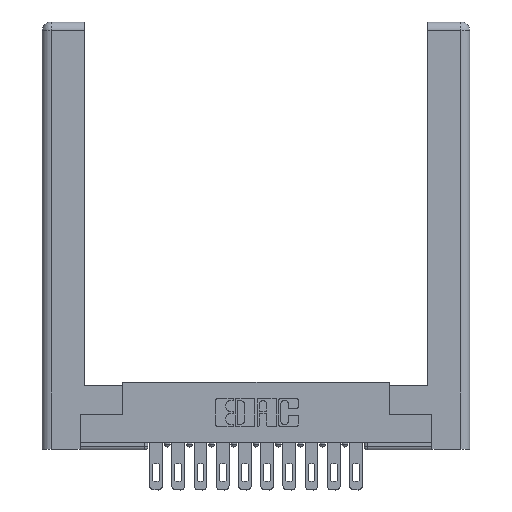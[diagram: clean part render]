
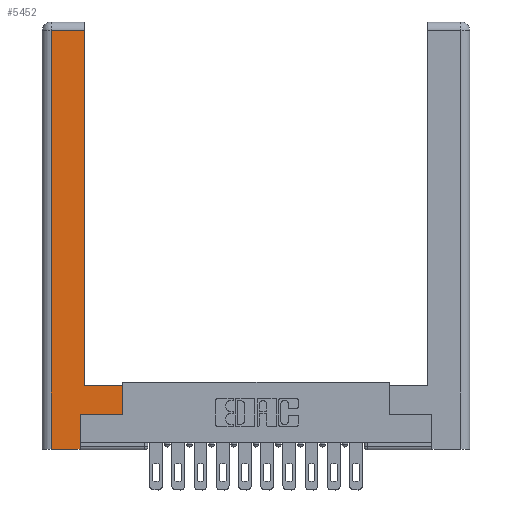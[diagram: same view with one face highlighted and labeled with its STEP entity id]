
A CAD part, top view. The second image highlights one B-rep face of the part: STEP entity #5452.
In plain terms, the highlighted planar face has unit normal (0, 0, 1).
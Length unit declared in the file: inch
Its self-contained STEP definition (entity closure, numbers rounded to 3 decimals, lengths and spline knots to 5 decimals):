
#91 = VERTEX_POINT ( 'NONE', #697 ) ;
#570 = VECTOR ( 'NONE', #2450, 39.37008 ) ;
#615 = DIRECTION ( 'NONE',  ( -1., 0., 0. ) ) ;
#697 = CARTESIAN_POINT ( 'NONE',  ( 0.0615, 2.94, 0. ) ) ;
#889 = CARTESIAN_POINT ( 'NONE',  ( 0.565, 0.45, 0. ) ) ;
#1073 = EDGE_CURVE ( 'NONE', #10897, #91, #7001, .T. ) ;
#1170 = VECTOR ( 'NONE', #13266, 39.37008 ) ;
#1200 = DIRECTION ( 'NONE',  ( -1., 0., 0. ) ) ;
#1414 = CARTESIAN_POINT ( 'NONE',  ( 0.295, 3., 0. ) ) ;
#1536 = ORIENTED_EDGE ( 'NONE', *, *, #7700, .T. ) ;
#1684 = FACE_OUTER_BOUND ( 'NONE', #1974, .T. ) ;
#1974 = EDGE_LOOP ( 'NONE', ( #2211, #2026, #6746, #7909, #13455, #1536, #10205, #5857 ) ) ;
#2026 = ORIENTED_EDGE ( 'NONE', *, *, #1073, .T. ) ;
#2033 = LINE ( 'NONE', #8176, #11463 ) ;
#2171 = VECTOR ( 'NONE', #4620, 39.37008 ) ;
#2211 = ORIENTED_EDGE ( 'NONE', *, *, #7150, .T. ) ;
#2450 = DIRECTION ( 'NONE',  ( -1., 0., 0. ) ) ;
#2715 = CARTESIAN_POINT ( 'NONE',  ( 0.295, 2.94, 0. ) ) ;
#2726 = VERTEX_POINT ( 'NONE', #13794 ) ;
#4239 = DIRECTION ( 'NONE',  ( 0., -1., 0. ) ) ;
#4620 = DIRECTION ( 'NONE',  ( 1., 0., 0. ) ) ;
#4949 = CARTESIAN_POINT ( 'NONE',  ( 0.265, 0., 0. ) ) ;
#5452 = ADVANCED_FACE ( 'NONE', ( #1684 ), #7741, .F. ) ;
#5709 = VERTEX_POINT ( 'NONE', #13240 ) ;
#5855 = CARTESIAN_POINT ( 'NONE',  ( 0.265, 0., 0. ) ) ;
#5857 = ORIENTED_EDGE ( 'NONE', *, *, #6094, .T. ) ;
#5921 = CARTESIAN_POINT ( 'NONE',  ( 0.0615, 2.94, 0. ) ) ;
#6094 = EDGE_CURVE ( 'NONE', #5709, #6208, #2033, .T. ) ;
#6208 = VERTEX_POINT ( 'NONE', #12914 ) ;
#6320 = VERTEX_POINT ( 'NONE', #14622 ) ;
#6377 = LINE ( 'NONE', #13341, #1170 ) ;
#6715 = VERTEX_POINT ( 'NONE', #4949 ) ;
#6746 = ORIENTED_EDGE ( 'NONE', *, *, #8407, .T. ) ;
#6782 = VECTOR ( 'NONE', #10089, 39.37008 ) ;
#7001 = LINE ( 'NONE', #5921, #570 ) ;
#7150 = EDGE_CURVE ( 'NONE', #6208, #10897, #10617, .T. ) ;
#7404 = EDGE_CURVE ( 'NONE', #9547, #6715, #13967, .T. ) ;
#7700 = EDGE_CURVE ( 'NONE', #2726, #6320, #6377, .T. ) ;
#7741 = PLANE ( 'NONE',  #7768 ) ;
#7768 = AXIS2_PLACEMENT_3D ( 'NONE', #8889, #13415, #615 ) ;
#7909 = ORIENTED_EDGE ( 'NONE', *, *, #7404, .T. ) ;
#8176 = CARTESIAN_POINT ( 'NONE',  ( 0.295, 0.45, 0. ) ) ;
#8407 = EDGE_CURVE ( 'NONE', #91, #9547, #12298, .T. ) ;
#8889 = CARTESIAN_POINT ( 'NONE',  ( 0., 0., 0. ) ) ;
#9465 = DIRECTION ( 'NONE',  ( 0., 1., 0. ) ) ;
#9547 = VERTEX_POINT ( 'NONE', #13936 ) ;
#10089 = DIRECTION ( 'NONE',  ( 0., 1., 0. ) ) ;
#10205 = ORIENTED_EDGE ( 'NONE', *, *, #14944, .T. ) ;
#10617 = LINE ( 'NONE', #1414, #15138 ) ;
#10897 = VERTEX_POINT ( 'NONE', #2715 ) ;
#11463 = VECTOR ( 'NONE', #1200, 39.37008 ) ;
#12298 = LINE ( 'NONE', #14669, #14143 ) ;
#12536 = LINE ( 'NONE', #889, #6782 ) ;
#12702 = CARTESIAN_POINT ( 'NONE',  ( 0.265, 0.245, 0. ) ) ;
#12914 = CARTESIAN_POINT ( 'NONE',  ( 0.295, 0.45, 0. ) ) ;
#13240 = CARTESIAN_POINT ( 'NONE',  ( 0.565, 0.45, 0. ) ) ;
#13266 = DIRECTION ( 'NONE',  ( 1., 0., 0. ) ) ;
#13341 = CARTESIAN_POINT ( 'NONE',  ( 0.565, 0.245, 0. ) ) ;
#13364 = VECTOR ( 'NONE', #15077, 39.37008 ) ;
#13415 = DIRECTION ( 'NONE',  ( 0., 0., -1. ) ) ;
#13455 = ORIENTED_EDGE ( 'NONE', *, *, #14576, .T. ) ;
#13794 = CARTESIAN_POINT ( 'NONE',  ( 0.265, 0.245, 0. ) ) ;
#13936 = CARTESIAN_POINT ( 'NONE',  ( 0.0615, 0., 0. ) ) ;
#13967 = LINE ( 'NONE', #5855, #2171 ) ;
#14085 = LINE ( 'NONE', #12702, #13364 ) ;
#14143 = VECTOR ( 'NONE', #4239, 39.37008 ) ;
#14576 = EDGE_CURVE ( 'NONE', #6715, #2726, #14085, .T. ) ;
#14622 = CARTESIAN_POINT ( 'NONE',  ( 0.565, 0.245, 0. ) ) ;
#14669 = CARTESIAN_POINT ( 'NONE',  ( 0.0615, 0., 0. ) ) ;
#14944 = EDGE_CURVE ( 'NONE', #6320, #5709, #12536, .T. ) ;
#15077 = DIRECTION ( 'NONE',  ( 0., 1., 0. ) ) ;
#15138 = VECTOR ( 'NONE', #9465, 39.37008 ) ;
